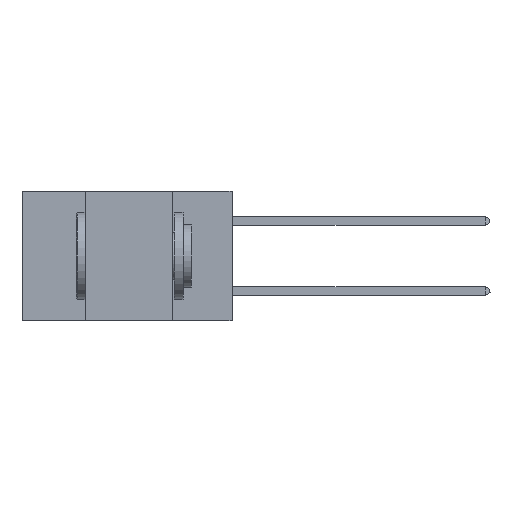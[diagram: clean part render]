
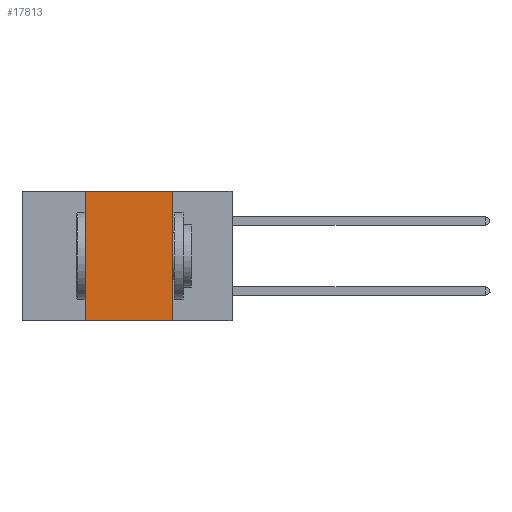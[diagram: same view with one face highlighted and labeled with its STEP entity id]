
A CAD part, left-side view. The second image highlights one B-rep face of the part: STEP entity #17813.
In plain terms, the highlighted planar face has unit normal (-1, 0, 0).
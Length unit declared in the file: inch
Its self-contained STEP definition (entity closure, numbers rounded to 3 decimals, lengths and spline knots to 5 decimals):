
#846 = DIRECTION ( 'NONE',  ( 1., 0., 0. ) ) ;
#2349 = LINE ( 'NONE', #32545, #35905 ) ;
#3132 = VECTOR ( 'NONE', #10023, 39.37008 ) ;
#4178 = FACE_OUTER_BOUND ( 'NONE', #9212, .T. ) ;
#5284 = EDGE_CURVE ( 'NONE', #36374, #7062, #18925, .T. ) ;
#6130 = VECTOR ( 'NONE', #25884, 39.37008 ) ;
#6753 = DIRECTION ( 'NONE',  ( 0., 0., -1. ) ) ;
#7014 = ORIENTED_EDGE ( 'NONE', *, *, #8590, .F. ) ;
#7062 = VERTEX_POINT ( 'NONE', #17516 ) ;
#7252 = LINE ( 'NONE', #33700, #23850 ) ;
#8096 = CARTESIAN_POINT ( 'NONE',  ( 0., 0.42, 0. ) ) ;
#8099 = ORIENTED_EDGE ( 'NONE', *, *, #14721, .F. ) ;
#8590 = EDGE_CURVE ( 'NONE', #8759, #14305, #2349, .T. ) ;
#8759 = VERTEX_POINT ( 'NONE', #14470 ) ;
#9212 = EDGE_LOOP ( 'NONE', ( #8099, #7014, #9215, #13429 ) ) ;
#9215 = ORIENTED_EDGE ( 'NONE', *, *, #16824, .F. ) ;
#10023 = DIRECTION ( 'NONE',  ( 0., -1., 0. ) ) ;
#12027 = PLANE ( 'NONE',  #28141 ) ;
#12935 = CARTESIAN_POINT ( 'NONE',  ( 0., 0.42, -0.37 ) ) ;
#13429 = ORIENTED_EDGE ( 'NONE', *, *, #5284, .T. ) ;
#14012 = LINE ( 'NONE', #8096, #6130 ) ;
#14305 = VERTEX_POINT ( 'NONE', #21587 ) ;
#14470 = CARTESIAN_POINT ( 'NONE',  ( 0., 0.42, 0. ) ) ;
#14721 = EDGE_CURVE ( 'NONE', #14305, #7062, #7252, .T. ) ;
#15013 = CARTESIAN_POINT ( 'NONE',  ( 0., 0.6, 0. ) ) ;
#15437 = CARTESIAN_POINT ( 'NONE',  ( 0., 0.6, -0.37 ) ) ;
#16824 = EDGE_CURVE ( 'NONE', #36374, #8759, #14012, .T. ) ;
#17516 = CARTESIAN_POINT ( 'NONE',  ( 0., 0.17, -0.37 ) ) ;
#17813 = ADVANCED_FACE ( 'NONE', ( #4178 ), #12027, .F. ) ;
#18925 = LINE ( 'NONE', #15437, #3132 ) ;
#21150 = DIRECTION ( 'NONE',  ( 0., -1., 0. ) ) ;
#21587 = CARTESIAN_POINT ( 'NONE',  ( 0., 0.17, 0. ) ) ;
#23850 = VECTOR ( 'NONE', #28491, 39.37008 ) ;
#25884 = DIRECTION ( 'NONE',  ( 0., 0., 1. ) ) ;
#28141 = AXIS2_PLACEMENT_3D ( 'NONE', #15013, #846, #6753 ) ;
#28491 = DIRECTION ( 'NONE',  ( 0., 0., -1. ) ) ;
#32545 = CARTESIAN_POINT ( 'NONE',  ( 0., 0.6, 0. ) ) ;
#33700 = CARTESIAN_POINT ( 'NONE',  ( 0., 0.17, 0. ) ) ;
#35905 = VECTOR ( 'NONE', #21150, 39.37008 ) ;
#36374 = VERTEX_POINT ( 'NONE', #12935 ) ;
